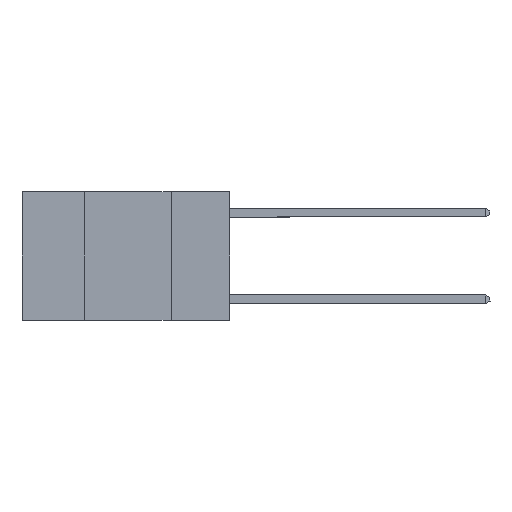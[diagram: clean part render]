
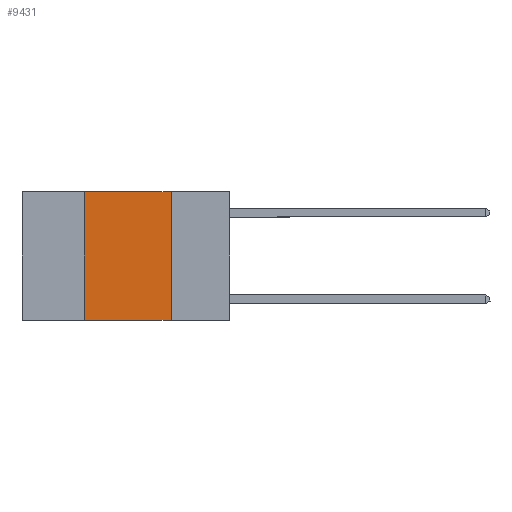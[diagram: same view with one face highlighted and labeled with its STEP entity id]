
A CAD part, left-side view. The second image highlights one B-rep face of the part: STEP entity #9431.
In plain terms, the highlighted planar face has unit normal (-1, 0, 0).
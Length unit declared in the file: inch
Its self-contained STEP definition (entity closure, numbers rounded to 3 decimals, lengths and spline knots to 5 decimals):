
#520 = VECTOR ( 'NONE', #1516, 39.37008 ) ;
#646 = PLANE ( 'NONE',  #2109 ) ;
#1011 = CARTESIAN_POINT ( 'NONE',  ( 0., 0.42, -0.37 ) ) ;
#1050 = DIRECTION ( 'NONE',  ( 0., -1., 0. ) ) ;
#1177 = EDGE_LOOP ( 'NONE', ( #3361, #1282, #3232, #2398 ) ) ;
#1282 = ORIENTED_EDGE ( 'NONE', *, *, #10029, .F. ) ;
#1516 = DIRECTION ( 'NONE',  ( 0., 0., -1. ) ) ;
#1641 = CARTESIAN_POINT ( 'NONE',  ( 0., 0.6, 0. ) ) ;
#1684 = DIRECTION ( 'NONE',  ( 1., 0., 0. ) ) ;
#1759 = VERTEX_POINT ( 'NONE', #1011 ) ;
#1873 = DIRECTION ( 'NONE',  ( 0., -1., 0. ) ) ;
#2109 = AXIS2_PLACEMENT_3D ( 'NONE', #1641, #1684, #8399 ) ;
#2398 = ORIENTED_EDGE ( 'NONE', *, *, #5659, .T. ) ;
#2771 = VECTOR ( 'NONE', #1873, 39.37008 ) ;
#3198 = LINE ( 'NONE', #3461, #520 ) ;
#3232 = ORIENTED_EDGE ( 'NONE', *, *, #3835, .F. ) ;
#3280 = VECTOR ( 'NONE', #1050, 39.37008 ) ;
#3361 = ORIENTED_EDGE ( 'NONE', *, *, #7001, .F. ) ;
#3461 = CARTESIAN_POINT ( 'NONE',  ( 0., 0.17, 0. ) ) ;
#3468 = CARTESIAN_POINT ( 'NONE',  ( 0., 0.17, -0.37 ) ) ;
#3835 = EDGE_CURVE ( 'NONE', #1759, #10045, #11026, .T. ) ;
#4211 = DIRECTION ( 'NONE',  ( 0., 0., 1. ) ) ;
#5659 = EDGE_CURVE ( 'NONE', #1759, #8844, #10438, .T. ) ;
#5937 = VECTOR ( 'NONE', #4211, 39.37008 ) ;
#6140 = CARTESIAN_POINT ( 'NONE',  ( 0., 0.42, 0. ) ) ;
#6307 = FACE_OUTER_BOUND ( 'NONE', #1177, .T. ) ;
#6398 = CARTESIAN_POINT ( 'NONE',  ( 0., 0.17, 0. ) ) ;
#6703 = CARTESIAN_POINT ( 'NONE',  ( 0., 0.6, -0.37 ) ) ;
#7001 = EDGE_CURVE ( 'NONE', #7048, #8844, #3198, .T. ) ;
#7048 = VERTEX_POINT ( 'NONE', #6398 ) ;
#7719 = CARTESIAN_POINT ( 'NONE',  ( 0., 0.6, 0. ) ) ;
#8399 = DIRECTION ( 'NONE',  ( 0., 0., -1. ) ) ;
#8844 = VERTEX_POINT ( 'NONE', #3468 ) ;
#8929 = LINE ( 'NONE', #7719, #3280 ) ;
#9431 = ADVANCED_FACE ( 'NONE', ( #6307 ), #646, .F. ) ;
#10029 = EDGE_CURVE ( 'NONE', #10045, #7048, #8929, .T. ) ;
#10045 = VERTEX_POINT ( 'NONE', #11654 ) ;
#10438 = LINE ( 'NONE', #6703, #2771 ) ;
#11026 = LINE ( 'NONE', #6140, #5937 ) ;
#11654 = CARTESIAN_POINT ( 'NONE',  ( 0., 0.42, 0. ) ) ;
